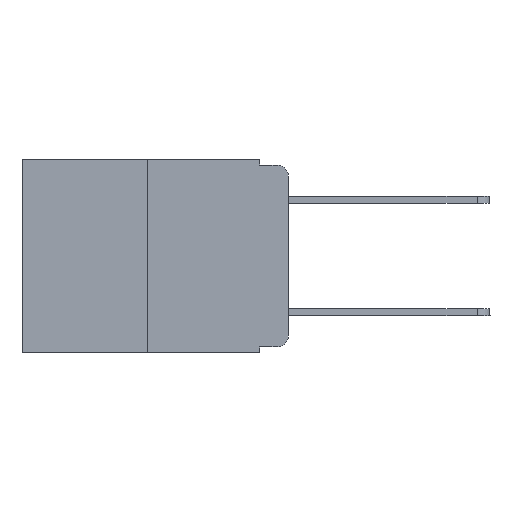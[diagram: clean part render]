
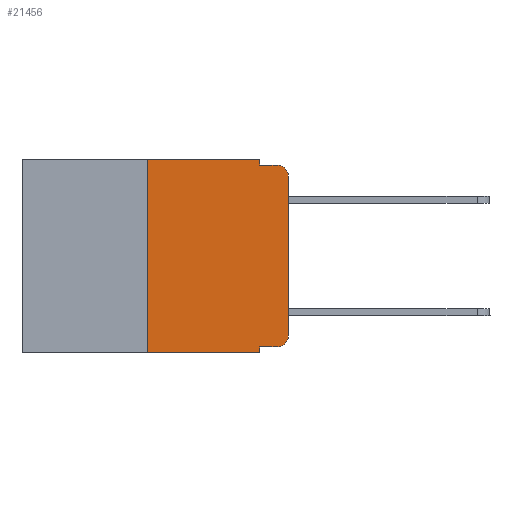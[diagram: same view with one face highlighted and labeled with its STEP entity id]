
A CAD part, left-side view. The second image highlights one B-rep face of the part: STEP entity #21456.
In plain terms, the highlighted planar face has unit normal (-1, 0, 0).
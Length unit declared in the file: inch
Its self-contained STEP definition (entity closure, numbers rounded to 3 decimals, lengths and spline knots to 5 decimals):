
#41 = LINE ( 'NONE', #9317, #1687 ) ;
#51 = VECTOR ( 'NONE', #9991, 39.37008 ) ;
#634 = EDGE_CURVE ( 'NONE', #6750, #6317, #14469, .T. ) ;
#702 = CARTESIAN_POINT ( 'NONE',  ( 0., 0.02, -0.03 ) ) ;
#789 = CARTESIAN_POINT ( 'NONE',  ( 0., 0.25, 0. ) ) ;
#1304 = VECTOR ( 'NONE', #8965, 39.37008 ) ;
#1315 = ORIENTED_EDGE ( 'NONE', *, *, #5033, .F. ) ;
#1687 = VECTOR ( 'NONE', #16960, 39.37008 ) ;
#1799 = EDGE_CURVE ( 'NONE', #15108, #20290, #17739, .T. ) ;
#1848 = CARTESIAN_POINT ( 'NONE',  ( 0., 0., -0.313 ) ) ;
#1964 = EDGE_CURVE ( 'NONE', #15108, #19032, #16352, .T. ) ;
#2097 = CIRCLE ( 'NONE', #11697, 0.02 ) ;
#2810 = CARTESIAN_POINT ( 'NONE',  ( 0., 0., 0. ) ) ;
#2817 = DIRECTION ( 'NONE',  ( 0., -1., 0. ) ) ;
#3241 = ORIENTED_EDGE ( 'NONE', *, *, #15907, .F. ) ;
#3305 = VERTEX_POINT ( 'NONE', #4953 ) ;
#3539 = PLANE ( 'NONE',  #20960 ) ;
#3860 = CARTESIAN_POINT ( 'NONE',  ( 0., 0.473, 0. ) ) ;
#4285 = EDGE_CURVE ( 'NONE', #6317, #18233, #16190, .T. ) ;
#4953 = CARTESIAN_POINT ( 'NONE',  ( 0., 0.02, -0.333 ) ) ;
#4963 = EDGE_LOOP ( 'NONE', ( #10529, #12061, #15634, #23213, #1315, #7442, #5260, #3241, #16795, #20778 ) ) ;
#5033 = EDGE_CURVE ( 'NONE', #19032, #7762, #21026, .T. ) ;
#5260 = ORIENTED_EDGE ( 'NONE', *, *, #1799, .T. ) ;
#5312 = CARTESIAN_POINT ( 'NONE',  ( 0., 0.25, 0. ) ) ;
#5411 = CARTESIAN_POINT ( 'NONE',  ( 0., 0., -0.03 ) ) ;
#5493 = DIRECTION ( 'NONE',  ( 0., 0., -1. ) ) ;
#5791 = DIRECTION ( 'NONE',  ( 1., 0., 0. ) ) ;
#6317 = VERTEX_POINT ( 'NONE', #5411 ) ;
#6573 = DIRECTION ( 'NONE',  ( 0., 0., -1. ) ) ;
#6750 = VERTEX_POINT ( 'NONE', #1848 ) ;
#7442 = ORIENTED_EDGE ( 'NONE', *, *, #1964, .F. ) ;
#7762 = VERTEX_POINT ( 'NONE', #15478 ) ;
#8040 = LINE ( 'NONE', #11822, #24558 ) ;
#8091 = CARTESIAN_POINT ( 'NONE',  ( 0., 0.473, -0.343 ) ) ;
#8909 = VECTOR ( 'NONE', #17328, 39.37008 ) ;
#8965 = DIRECTION ( 'NONE',  ( 0., 0., 1. ) ) ;
#9317 = CARTESIAN_POINT ( 'NONE',  ( 0., 0.051, 0. ) ) ;
#9398 = AXIS2_PLACEMENT_3D ( 'NONE', #702, #16096, #6573 ) ;
#9991 = DIRECTION ( 'NONE',  ( 0., -1., 0. ) ) ;
#10069 = CARTESIAN_POINT ( 'NONE',  ( 0., 0.051, -0.343 ) ) ;
#10260 = CARTESIAN_POINT ( 'NONE',  ( 0., 0.25, -0.343 ) ) ;
#10529 = ORIENTED_EDGE ( 'NONE', *, *, #634, .T. ) ;
#11198 = CARTESIAN_POINT ( 'NONE',  ( 0., 0.473, 0. ) ) ;
#11370 = VECTOR ( 'NONE', #22092, 39.37008 ) ;
#11697 = AXIS2_PLACEMENT_3D ( 'NONE', #15034, #22650, #5493 ) ;
#11822 = CARTESIAN_POINT ( 'NONE',  ( 0., 0.051, 0. ) ) ;
#12061 = ORIENTED_EDGE ( 'NONE', *, *, #4285, .T. ) ;
#12672 = VERTEX_POINT ( 'NONE', #15184 ) ;
#12941 = VECTOR ( 'NONE', #13142, 39.37008 ) ;
#13142 = DIRECTION ( 'NONE',  ( 0., -1., 0. ) ) ;
#13451 = DIRECTION ( 'NONE',  ( 0., 0., -1. ) ) ;
#14469 = LINE ( 'NONE', #2810, #11370 ) ;
#14843 = EDGE_CURVE ( 'NONE', #12672, #3305, #18661, .T. ) ;
#15034 = CARTESIAN_POINT ( 'NONE',  ( 0., 0.02, -0.313 ) ) ;
#15108 = VERTEX_POINT ( 'NONE', #10260 ) ;
#15125 = CARTESIAN_POINT ( 'NONE',  ( 0., 0.051, -0.01 ) ) ;
#15184 = CARTESIAN_POINT ( 'NONE',  ( 0., 0.051, -0.333 ) ) ;
#15195 = CARTESIAN_POINT ( 'NONE',  ( 0., 0.051, -0.01 ) ) ;
#15478 = CARTESIAN_POINT ( 'NONE',  ( 0., 0.051, 0. ) ) ;
#15634 = ORIENTED_EDGE ( 'NONE', *, *, #15847, .F. ) ;
#15674 = DIRECTION ( 'NONE',  ( 0., 0., -1. ) ) ;
#15847 = EDGE_CURVE ( 'NONE', #20482, #18233, #18832, .T. ) ;
#15907 = EDGE_CURVE ( 'NONE', #12672, #20290, #41, .T. ) ;
#16096 = DIRECTION ( 'NONE',  ( -1., 0., 0. ) ) ;
#16190 = CIRCLE ( 'NONE', #9398, 0.02 ) ;
#16207 = EDGE_CURVE ( 'NONE', #3305, #6750, #2097, .T. ) ;
#16278 = CARTESIAN_POINT ( 'NONE',  ( 0., 0.02, -0.01 ) ) ;
#16352 = LINE ( 'NONE', #5312, #1304 ) ;
#16516 = VECTOR ( 'NONE', #2817, 39.37008 ) ;
#16771 = CARTESIAN_POINT ( 'NONE',  ( 0., 0.051, -0.333 ) ) ;
#16795 = ORIENTED_EDGE ( 'NONE', *, *, #14843, .T. ) ;
#16960 = DIRECTION ( 'NONE',  ( 0., 0., -1. ) ) ;
#17073 = FACE_OUTER_BOUND ( 'NONE', #4963, .T. ) ;
#17328 = DIRECTION ( 'NONE',  ( 0., -1., 0. ) ) ;
#17616 = EDGE_CURVE ( 'NONE', #7762, #20482, #8040, .T. ) ;
#17739 = LINE ( 'NONE', #8091, #16516 ) ;
#18233 = VERTEX_POINT ( 'NONE', #16278 ) ;
#18661 = LINE ( 'NONE', #16771, #12941 ) ;
#18832 = LINE ( 'NONE', #15195, #8909 ) ;
#19032 = VERTEX_POINT ( 'NONE', #789 ) ;
#20290 = VERTEX_POINT ( 'NONE', #10069 ) ;
#20482 = VERTEX_POINT ( 'NONE', #15125 ) ;
#20778 = ORIENTED_EDGE ( 'NONE', *, *, #16207, .T. ) ;
#20960 = AXIS2_PLACEMENT_3D ( 'NONE', #11198, #5791, #13451 ) ;
#21026 = LINE ( 'NONE', #3860, #51 ) ;
#21456 = ADVANCED_FACE ( 'NONE', ( #17073 ), #3539, .F. ) ;
#22092 = DIRECTION ( 'NONE',  ( 0., 0., 1. ) ) ;
#22650 = DIRECTION ( 'NONE',  ( -1., 0., 0. ) ) ;
#23213 = ORIENTED_EDGE ( 'NONE', *, *, #17616, .F. ) ;
#24558 = VECTOR ( 'NONE', #15674, 39.37008 ) ;
